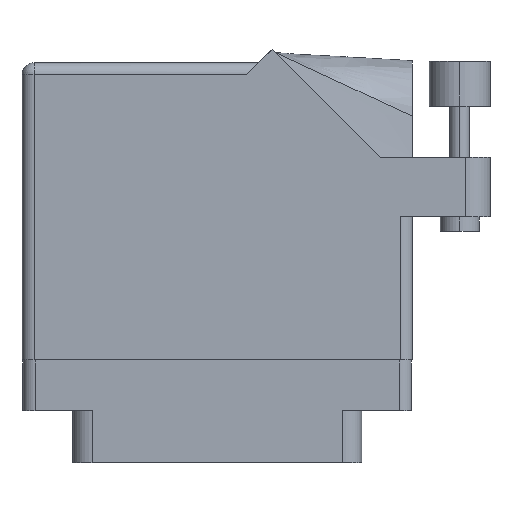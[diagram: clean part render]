
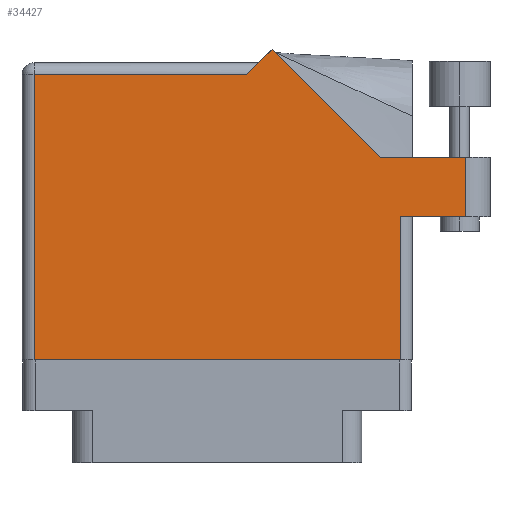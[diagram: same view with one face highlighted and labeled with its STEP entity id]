
A CAD part, front view. The second image highlights one B-rep face of the part: STEP entity #34427.
In plain terms, the highlighted face is planar.
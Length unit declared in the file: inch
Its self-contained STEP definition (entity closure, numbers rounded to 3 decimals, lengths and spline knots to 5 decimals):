
#297 = FACE_OUTER_BOUND ( 'NONE', #32648, .T. ) ;
#705 = ORIENTED_EDGE ( 'NONE', *, *, #14413, .T. ) ;
#1058 = VERTEX_POINT ( 'NONE', #3233 ) ;
#1415 = LINE ( 'NONE', #6880, #4726 ) ;
#2057 = DIRECTION ( 'NONE',  ( 0., 1., 0. ) ) ;
#3002 = AXIS2_PLACEMENT_3D ( 'NONE', #5411, #16190, #5583 ) ;
#3233 = CARTESIAN_POINT ( 'NONE',  ( 1.155, 1.468, 0. ) ) ;
#3576 = EDGE_CURVE ( 'NONE', #27410, #24559, #15343, .T. ) ;
#3634 = ORIENTED_EDGE ( 'NONE', *, *, #3576, .T. ) ;
#3918 = VECTOR ( 'NONE', #29928, 39.37008 ) ;
#4422 = VECTOR ( 'NONE', #30102, 39.37008 ) ;
#4581 = DIRECTION ( 'NONE',  ( -0.707, -0.707, 0. ) ) ;
#4725 = LINE ( 'NONE', #19626, #6234 ) ;
#4726 = VECTOR ( 'NONE', #4581, 39.37008 ) ;
#4823 = CARTESIAN_POINT ( 'NONE',  ( 1.948, 0.737, 0. ) ) ;
#4831 = DIRECTION ( 'NONE',  ( -1., 0., 0. ) ) ;
#5411 = CARTESIAN_POINT ( 'NONE',  ( 0., 1.53, 0. ) ) ;
#5583 = DIRECTION ( 'NONE',  ( -1., 0., 0. ) ) ;
#6234 = VECTOR ( 'NONE', #2057, 39.37008 ) ;
#6830 = CARTESIAN_POINT ( 'NONE',  ( 0.062, 1.468, 0. ) ) ;
#6880 = CARTESIAN_POINT ( 'NONE',  ( 1.217, 1.53, 0. ) ) ;
#7184 = EDGE_CURVE ( 'NONE', #17897, #19094, #11187, .T. ) ;
#8269 = VECTOR ( 'NONE', #17934, 39.37008 ) ;
#8358 = CARTESIAN_POINT ( 'NONE',  ( 2.285, 1.044, 0. ) ) ;
#8518 = ORIENTED_EDGE ( 'NONE', *, *, #19111, .T. ) ;
#9342 = CARTESIAN_POINT ( 'NONE',  ( 1.84442, 1.044, 0. ) ) ;
#9749 = CARTESIAN_POINT ( 'NONE',  ( 1.28771, 1.60071, 0. ) ) ;
#10237 = ORIENTED_EDGE ( 'NONE', *, *, #31204, .T. ) ;
#11187 = LINE ( 'NONE', #29923, #4422 ) ;
#11188 = ORIENTED_EDGE ( 'NONE', *, *, #31111, .T. ) ;
#12394 = LINE ( 'NONE', #20030, #29303 ) ;
#13587 = CARTESIAN_POINT ( 'NONE',  ( 1.948, 0., 0. ) ) ;
#14413 = EDGE_CURVE ( 'NONE', #1058, #27858, #26360, .T. ) ;
#15152 = EDGE_CURVE ( 'NONE', #27858, #23967, #31372, .T. ) ;
#15343 = LINE ( 'NONE', #9342, #16034 ) ;
#15536 = VECTOR ( 'NONE', #26193, 39.37008 ) ;
#15577 = ORIENTED_EDGE ( 'NONE', *, *, #28647, .T. ) ;
#16034 = VECTOR ( 'NONE', #22932, 39.37008 ) ;
#16190 = DIRECTION ( 'NONE',  ( 0., 0., -1. ) ) ;
#17897 = VERTEX_POINT ( 'NONE', #4823 ) ;
#17934 = DIRECTION ( 'NONE',  ( 0., -1., 0. ) ) ;
#18045 = ORIENTED_EDGE ( 'NONE', *, *, #7184, .T. ) ;
#19094 = VERTEX_POINT ( 'NONE', #29998 ) ;
#19111 = EDGE_CURVE ( 'NONE', #28197, #27410, #28662, .T. ) ;
#19626 = CARTESIAN_POINT ( 'NONE',  ( 1.948, 0.737, 0. ) ) ;
#19855 = ORIENTED_EDGE ( 'NONE', *, *, #30342, .T. ) ;
#20030 = CARTESIAN_POINT ( 'NONE',  ( 0., 0., 0. ) ) ;
#21419 = CARTESIAN_POINT ( 'NONE',  ( 0., 1.468, 0. ) ) ;
#22282 = ORIENTED_EDGE ( 'NONE', *, *, #15152, .T. ) ;
#22932 = DIRECTION ( 'NONE',  ( -0.707, 0.707, 0. ) ) ;
#23967 = VERTEX_POINT ( 'NONE', #27483 ) ;
#24309 = PLANE ( 'NONE',  #3002 ) ;
#24559 = VERTEX_POINT ( 'NONE', #9749 ) ;
#26193 = DIRECTION ( 'NONE',  ( -1., 0., 0. ) ) ;
#26296 = CARTESIAN_POINT ( 'NONE',  ( 1.84442, 1.044, 0. ) ) ;
#26360 = LINE ( 'NONE', #21419, #15536 ) ;
#27410 = VERTEX_POINT ( 'NONE', #26296 ) ;
#27483 = CARTESIAN_POINT ( 'NONE',  ( 0.062, 0., 0. ) ) ;
#27858 = VERTEX_POINT ( 'NONE', #6830 ) ;
#28197 = VERTEX_POINT ( 'NONE', #33654 ) ;
#28483 = DIRECTION ( 'NONE',  ( 1., 0., 0. ) ) ;
#28538 = CARTESIAN_POINT ( 'NONE',  ( 0.062, 0., 0. ) ) ;
#28647 = EDGE_CURVE ( 'NONE', #24559, #1058, #1415, .T. ) ;
#28662 = LINE ( 'NONE', #29028, #29193 ) ;
#28870 = VERTEX_POINT ( 'NONE', #13587 ) ;
#29028 = CARTESIAN_POINT ( 'NONE',  ( 2.41, 1.044, 0. ) ) ;
#29193 = VECTOR ( 'NONE', #4831, 39.37008 ) ;
#29303 = VECTOR ( 'NONE', #28483, 39.37008 ) ;
#29923 = CARTESIAN_POINT ( 'NONE',  ( 2.01, 0.737, 0. ) ) ;
#29928 = DIRECTION ( 'NONE',  ( 0., 1., 0. ) ) ;
#29998 = CARTESIAN_POINT ( 'NONE',  ( 2.285, 0.737, 0. ) ) ;
#30102 = DIRECTION ( 'NONE',  ( 1., 0., 0. ) ) ;
#30342 = EDGE_CURVE ( 'NONE', #28870, #17897, #4725, .T. ) ;
#31111 = EDGE_CURVE ( 'NONE', #19094, #28197, #33102, .T. ) ;
#31204 = EDGE_CURVE ( 'NONE', #23967, #28870, #12394, .T. ) ;
#31372 = LINE ( 'NONE', #28538, #8269 ) ;
#32648 = EDGE_LOOP ( 'NONE', ( #18045, #11188, #8518, #3634, #15577, #705, #22282, #10237, #19855 ) ) ;
#33102 = LINE ( 'NONE', #8358, #3918 ) ;
#33654 = CARTESIAN_POINT ( 'NONE',  ( 2.285, 1.044, 0. ) ) ;
#34427 = ADVANCED_FACE ( 'NONE', ( #297 ), #24309, .F. ) ;
